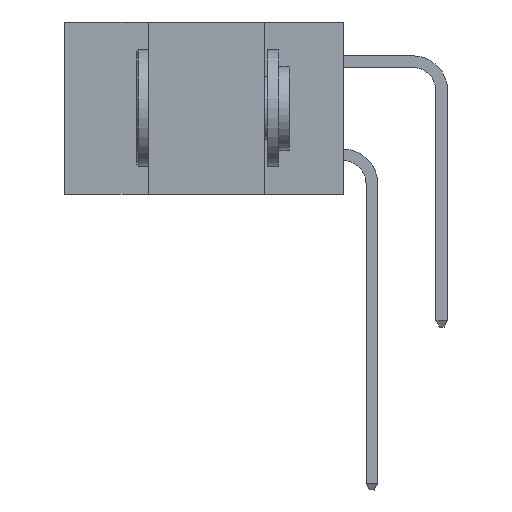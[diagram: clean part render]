
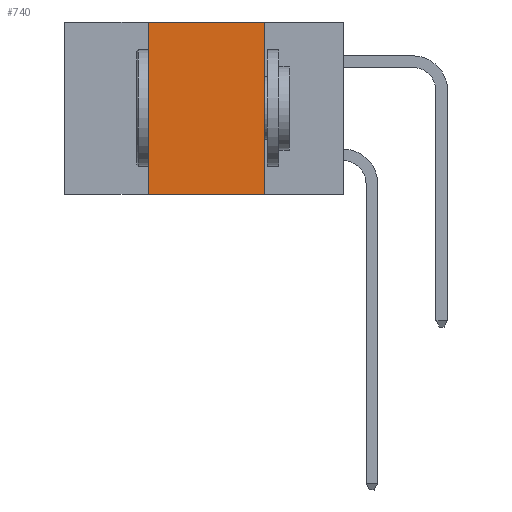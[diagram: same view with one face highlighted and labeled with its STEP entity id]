
A CAD part, left-side view. The second image highlights one B-rep face of the part: STEP entity #740.
In plain terms, the highlighted planar face has unit normal (-1, 0, 0).
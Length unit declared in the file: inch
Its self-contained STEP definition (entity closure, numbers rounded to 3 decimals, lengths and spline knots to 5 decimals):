
#740 = ADVANCED_FACE ( 'NONE', ( #30534 ), #24866, .F. ) ;
#914 = EDGE_CURVE ( 'NONE', #24758, #4266, #8724, .T. ) ;
#2942 = EDGE_LOOP ( 'NONE', ( #29094, #29177, #3336, #4304 ) ) ;
#3302 = CARTESIAN_POINT ( 'NONE',  ( 0., 0.6, 0. ) ) ;
#3336 = ORIENTED_EDGE ( 'NONE', *, *, #20362, .F. ) ;
#4004 = VECTOR ( 'NONE', #7080, 39.37008 ) ;
#4209 = CARTESIAN_POINT ( 'NONE',  ( 0., 0.42, -0.37 ) ) ;
#4266 = VERTEX_POINT ( 'NONE', #25747 ) ;
#4304 = ORIENTED_EDGE ( 'NONE', *, *, #16123, .T. ) ;
#5258 = LINE ( 'NONE', #29658, #19321 ) ;
#5726 = AXIS2_PLACEMENT_3D ( 'NONE', #7921, #10509, #17719 ) ;
#6979 = CARTESIAN_POINT ( 'NONE',  ( 0., 0.42, 0. ) ) ;
#7080 = DIRECTION ( 'NONE',  ( 0., 0., 1. ) ) ;
#7921 = CARTESIAN_POINT ( 'NONE',  ( 0., 0.6, 0. ) ) ;
#8208 = DIRECTION ( 'NONE',  ( 0., -1., 0. ) ) ;
#8724 = LINE ( 'NONE', #20506, #18302 ) ;
#8862 = DIRECTION ( 'NONE',  ( 0., 0., -1. ) ) ;
#10509 = DIRECTION ( 'NONE',  ( 1., 0., 0. ) ) ;
#16085 = EDGE_CURVE ( 'NONE', #26710, #24758, #23069, .T. ) ;
#16123 = EDGE_CURVE ( 'NONE', #19908, #4266, #5258, .T. ) ;
#17719 = DIRECTION ( 'NONE',  ( 0., 0., -1. ) ) ;
#18302 = VECTOR ( 'NONE', #8862, 39.37008 ) ;
#19321 = VECTOR ( 'NONE', #8208, 39.37008 ) ;
#19908 = VERTEX_POINT ( 'NONE', #4209 ) ;
#20362 = EDGE_CURVE ( 'NONE', #19908, #26710, #29536, .T. ) ;
#20506 = CARTESIAN_POINT ( 'NONE',  ( 0., 0.17, 0. ) ) ;
#21554 = CARTESIAN_POINT ( 'NONE',  ( 0., 0.42, 0. ) ) ;
#23069 = LINE ( 'NONE', #3302, #27087 ) ;
#24758 = VERTEX_POINT ( 'NONE', #30459 ) ;
#24866 = PLANE ( 'NONE',  #5726 ) ;
#25747 = CARTESIAN_POINT ( 'NONE',  ( 0., 0.17, -0.37 ) ) ;
#26710 = VERTEX_POINT ( 'NONE', #21554 ) ;
#26995 = DIRECTION ( 'NONE',  ( 0., -1., 0. ) ) ;
#27087 = VECTOR ( 'NONE', #26995, 39.37008 ) ;
#29094 = ORIENTED_EDGE ( 'NONE', *, *, #914, .F. ) ;
#29177 = ORIENTED_EDGE ( 'NONE', *, *, #16085, .F. ) ;
#29536 = LINE ( 'NONE', #6979, #4004 ) ;
#29658 = CARTESIAN_POINT ( 'NONE',  ( 0., 0.6, -0.37 ) ) ;
#30459 = CARTESIAN_POINT ( 'NONE',  ( 0., 0.17, 0. ) ) ;
#30534 = FACE_OUTER_BOUND ( 'NONE', #2942, .T. ) ;
